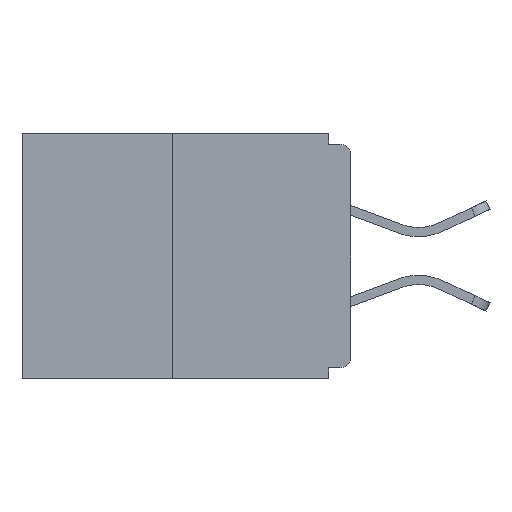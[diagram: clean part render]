
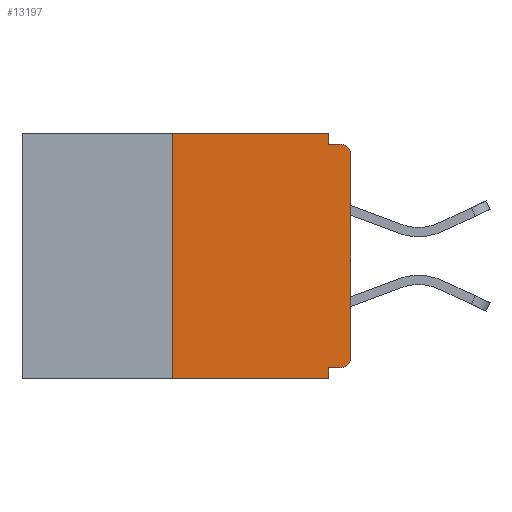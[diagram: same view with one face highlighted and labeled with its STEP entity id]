
A CAD part, left-side view. The second image highlights one B-rep face of the part: STEP entity #13197.
In plain terms, the highlighted planar face has unit normal (-1, 0, 0).
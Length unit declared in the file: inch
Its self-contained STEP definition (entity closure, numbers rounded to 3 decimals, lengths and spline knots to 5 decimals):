
#106 = DIRECTION ( 'NONE',  ( 0., 0., -1. ) ) ;
#979 = ORIENTED_EDGE ( 'NONE', *, *, #9656, .F. ) ;
#1044 = CARTESIAN_POINT ( 'NONE',  ( 0., 0.46, 0. ) ) ;
#1106 = LINE ( 'NONE', #22999, #24751 ) ;
#1273 = DIRECTION ( 'NONE',  ( 0., -1., 0. ) ) ;
#1304 = VERTEX_POINT ( 'NONE', #1320 ) ;
#1320 = CARTESIAN_POINT ( 'NONE',  ( 0., 0.015, -0.015 ) ) ;
#1610 = EDGE_CURVE ( 'NONE', #13485, #2690, #12151, .T. ) ;
#2176 = EDGE_CURVE ( 'NONE', #13358, #25654, #2214, .T. ) ;
#2214 = LINE ( 'NONE', #19819, #5288 ) ;
#2276 = CARTESIAN_POINT ( 'NONE',  ( 0., 0., -0.313 ) ) ;
#2317 = DIRECTION ( 'NONE',  ( 0., 0., -1. ) ) ;
#2459 = CARTESIAN_POINT ( 'NONE',  ( 0., 0., -0.03 ) ) ;
#2690 = VERTEX_POINT ( 'NONE', #26437 ) ;
#2717 = DIRECTION ( 'NONE',  ( 0., 0., -1. ) ) ;
#3420 = FACE_OUTER_BOUND ( 'NONE', #18471, .T. ) ;
#3448 = CARTESIAN_POINT ( 'NONE',  ( 0., 0.25, -0.343 ) ) ;
#3483 = CIRCLE ( 'NONE', #25675, 0.015 ) ;
#3559 = CARTESIAN_POINT ( 'NONE',  ( 0., 0.031, -0.015 ) ) ;
#4340 = CARTESIAN_POINT ( 'NONE',  ( 0., 0.015, -0.03 ) ) ;
#4663 = VECTOR ( 'NONE', #22735, 39.37008 ) ;
#4836 = CARTESIAN_POINT ( 'NONE',  ( 0., 0.25, 0. ) ) ;
#5288 = VECTOR ( 'NONE', #15607, 39.37008 ) ;
#6986 = VERTEX_POINT ( 'NONE', #2459 ) ;
#7071 = AXIS2_PLACEMENT_3D ( 'NONE', #1044, #20832, #7370 ) ;
#7242 = EDGE_CURVE ( 'NONE', #2690, #25654, #23603, .T. ) ;
#7333 = VECTOR ( 'NONE', #1273, 39.37008 ) ;
#7370 = DIRECTION ( 'NONE',  ( 0., 0., -1. ) ) ;
#7558 = PLANE ( 'NONE',  #7071 ) ;
#7718 = ORIENTED_EDGE ( 'NONE', *, *, #15266, .F. ) ;
#7789 = DIRECTION ( 'NONE',  ( 0., 0., -1. ) ) ;
#9205 = ORIENTED_EDGE ( 'NONE', *, *, #25643, .T. ) ;
#9654 = CARTESIAN_POINT ( 'NONE',  ( 0., 0.031, 0. ) ) ;
#9656 = EDGE_CURVE ( 'NONE', #22354, #16363, #26252, .T. ) ;
#9895 = EDGE_CURVE ( 'NONE', #11419, #22354, #27606, .T. ) ;
#11419 = VERTEX_POINT ( 'NONE', #4836 ) ;
#11661 = EDGE_CURVE ( 'NONE', #18741, #6986, #1106, .T. ) ;
#12151 = LINE ( 'NONE', #15919, #4663 ) ;
#12517 = CARTESIAN_POINT ( 'NONE',  ( 0., 0.25, 0. ) ) ;
#12701 = DIRECTION ( 'NONE',  ( 0., 0., 1. ) ) ;
#13018 = DIRECTION ( 'NONE',  ( -1., 0., 0. ) ) ;
#13136 = LINE ( 'NONE', #16544, #7333 ) ;
#13197 = ADVANCED_FACE ( 'NONE', ( #3420 ), #7558, .F. ) ;
#13272 = LINE ( 'NONE', #12517, #19430 ) ;
#13358 = VERTEX_POINT ( 'NONE', #3448 ) ;
#13378 = CARTESIAN_POINT ( 'NONE',  ( 0., 0.031, -0.343 ) ) ;
#13485 = VERTEX_POINT ( 'NONE', #17389 ) ;
#13702 = CARTESIAN_POINT ( 'NONE',  ( 0., 0.031, 0. ) ) ;
#14730 = CARTESIAN_POINT ( 'NONE',  ( 0., 0.46, 0. ) ) ;
#15266 = EDGE_CURVE ( 'NONE', #13358, #11419, #13272, .T. ) ;
#15607 = DIRECTION ( 'NONE',  ( 0., -1., 0. ) ) ;
#15919 = CARTESIAN_POINT ( 'NONE',  ( 0., 0., -0.328 ) ) ;
#16363 = VERTEX_POINT ( 'NONE', #3559 ) ;
#16454 = DIRECTION ( 'NONE',  ( 0., 0., 1. ) ) ;
#16544 = CARTESIAN_POINT ( 'NONE',  ( 0., 0., -0.015 ) ) ;
#16897 = CIRCLE ( 'NONE', #21025, 0.015 ) ;
#17389 = CARTESIAN_POINT ( 'NONE',  ( 0., 0.015, -0.328 ) ) ;
#17523 = CARTESIAN_POINT ( 'NONE',  ( 0., 0.015, -0.313 ) ) ;
#17577 = ORIENTED_EDGE ( 'NONE', *, *, #23745, .F. ) ;
#17917 = ORIENTED_EDGE ( 'NONE', *, *, #7242, .F. ) ;
#17979 = ORIENTED_EDGE ( 'NONE', *, *, #11661, .T. ) ;
#18471 = EDGE_LOOP ( 'NONE', ( #18563, #7718, #27929, #17917, #19296, #23118, #17979, #9205, #17577, #979 ) ) ;
#18563 = ORIENTED_EDGE ( 'NONE', *, *, #9895, .F. ) ;
#18741 = VERTEX_POINT ( 'NONE', #2276 ) ;
#18926 = DIRECTION ( 'NONE',  ( 0., -1., 0. ) ) ;
#19296 = ORIENTED_EDGE ( 'NONE', *, *, #1610, .F. ) ;
#19430 = VECTOR ( 'NONE', #12701, 39.37008 ) ;
#19819 = CARTESIAN_POINT ( 'NONE',  ( 0., 0.46, -0.343 ) ) ;
#20832 = DIRECTION ( 'NONE',  ( 1., 0., 0. ) ) ;
#21025 = AXIS2_PLACEMENT_3D ( 'NONE', #4340, #26616, #2317 ) ;
#21739 = VECTOR ( 'NONE', #18926, 39.37008 ) ;
#21767 = VECTOR ( 'NONE', #2717, 39.37008 ) ;
#22354 = VERTEX_POINT ( 'NONE', #9654 ) ;
#22735 = DIRECTION ( 'NONE',  ( 0., 1., 0. ) ) ;
#22999 = CARTESIAN_POINT ( 'NONE',  ( 0., 0., 0. ) ) ;
#23118 = ORIENTED_EDGE ( 'NONE', *, *, #27513, .T. ) ;
#23603 = LINE ( 'NONE', #25207, #25672 ) ;
#23745 = EDGE_CURVE ( 'NONE', #16363, #1304, #13136, .T. ) ;
#24751 = VECTOR ( 'NONE', #16454, 39.37008 ) ;
#25207 = CARTESIAN_POINT ( 'NONE',  ( 0., 0.031, -0.343 ) ) ;
#25643 = EDGE_CURVE ( 'NONE', #6986, #1304, #16897, .T. ) ;
#25654 = VERTEX_POINT ( 'NONE', #13378 ) ;
#25672 = VECTOR ( 'NONE', #7789, 39.37008 ) ;
#25675 = AXIS2_PLACEMENT_3D ( 'NONE', #17523, #13018, #106 ) ;
#26252 = LINE ( 'NONE', #13702, #21767 ) ;
#26437 = CARTESIAN_POINT ( 'NONE',  ( 0., 0.031, -0.328 ) ) ;
#26616 = DIRECTION ( 'NONE',  ( -1., 0., 0. ) ) ;
#27513 = EDGE_CURVE ( 'NONE', #13485, #18741, #3483, .T. ) ;
#27606 = LINE ( 'NONE', #14730, #21739 ) ;
#27929 = ORIENTED_EDGE ( 'NONE', *, *, #2176, .T. ) ;
